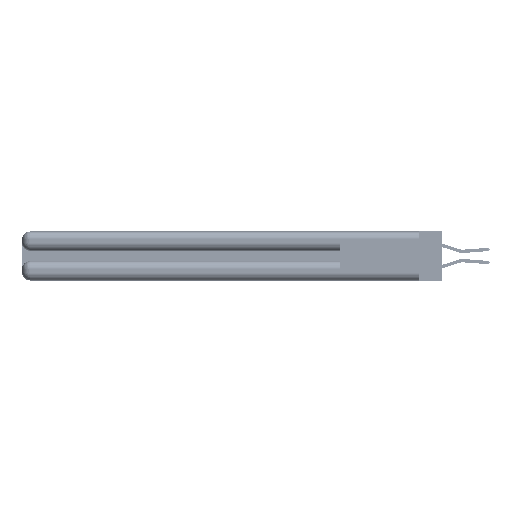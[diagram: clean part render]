
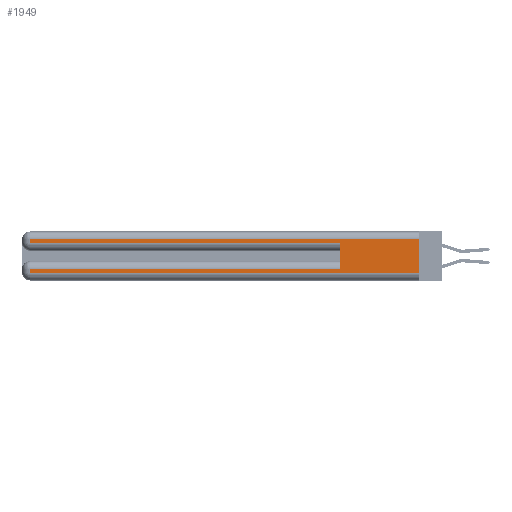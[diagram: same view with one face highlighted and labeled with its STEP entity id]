
A CAD part, left-side view. The second image highlights one B-rep face of the part: STEP entity #1949.
In plain terms, the highlighted planar face has unit normal (-1, 0, 0).
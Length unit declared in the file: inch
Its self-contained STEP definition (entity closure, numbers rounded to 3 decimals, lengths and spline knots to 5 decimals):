
#197 = VECTOR ( 'NONE', #21409, 39.37008 ) ;
#849 = CARTESIAN_POINT ( 'NONE',  ( 0., 0.6, 0.145 ) ) ;
#1949 = ADVANCED_FACE ( 'NONE', ( #14343 ), #17856, .F. ) ;
#2125 = CARTESIAN_POINT ( 'NONE',  ( 0., 0., 0.06 ) ) ;
#2189 = EDGE_CURVE ( 'NONE', #31588, #5667, #36107, .T. ) ;
#2326 = DIRECTION ( 'NONE',  ( 0., 0., -1. ) ) ;
#3190 = CARTESIAN_POINT ( 'NONE',  ( 0., 0., 0.31 ) ) ;
#3318 = EDGE_CURVE ( 'NONE', #8492, #39988, #34006, .T. ) ;
#4852 = AXIS2_PLACEMENT_3D ( 'NONE', #13588, #9310, #22088 ) ;
#4855 = VECTOR ( 'NONE', #26163, 39.37008 ) ;
#5667 = VERTEX_POINT ( 'NONE', #52385 ) ;
#6557 = EDGE_CURVE ( 'NONE', #14769, #17361, #39207, .T. ) ;
#6794 = EDGE_CURVE ( 'NONE', #20744, #17361, #37201, .T. ) ;
#6870 = LINE ( 'NONE', #19288, #27984 ) ;
#8383 = EDGE_CURVE ( 'NONE', #20744, #12990, #44927, .T. ) ;
#8492 = VERTEX_POINT ( 'NONE', #11783 ) ;
#9310 = DIRECTION ( 'NONE',  ( 1., 0., 0. ) ) ;
#9988 = LINE ( 'NONE', #36077, #31182 ) ;
#10097 = LINE ( 'NONE', #12913, #197 ) ;
#11430 = ORIENTED_EDGE ( 'NONE', *, *, #38793, .T. ) ;
#11783 = CARTESIAN_POINT ( 'NONE',  ( 0., 0., 0.31 ) ) ;
#12913 = CARTESIAN_POINT ( 'NONE',  ( 0., 2.94, 0.37 ) ) ;
#12958 = EDGE_CURVE ( 'NONE', #39988, #14769, #10097, .T. ) ;
#12990 = VERTEX_POINT ( 'NONE', #42606 ) ;
#13499 = ORIENTED_EDGE ( 'NONE', *, *, #2189, .T. ) ;
#13588 = CARTESIAN_POINT ( 'NONE',  ( 0., 0., 0.37 ) ) ;
#14061 = ORIENTED_EDGE ( 'NONE', *, *, #12958, .T. ) ;
#14343 = FACE_OUTER_BOUND ( 'NONE', #54278, .T. ) ;
#14769 = VERTEX_POINT ( 'NONE', #50677 ) ;
#15781 = CARTESIAN_POINT ( 'NONE',  ( 0., 2.94, 0.31 ) ) ;
#16213 = CARTESIAN_POINT ( 'NONE',  ( 0., 0., 0.285 ) ) ;
#17361 = VERTEX_POINT ( 'NONE', #48994 ) ;
#17856 = PLANE ( 'NONE',  #4852 ) ;
#19288 = CARTESIAN_POINT ( 'NONE',  ( 0., 2.94, 0.37 ) ) ;
#20197 = ORIENTED_EDGE ( 'NONE', *, *, #8383, .T. ) ;
#20744 = VERTEX_POINT ( 'NONE', #27229 ) ;
#21409 = DIRECTION ( 'NONE',  ( 0., 0., -1. ) ) ;
#22088 = DIRECTION ( 'NONE',  ( 0., 0., -1. ) ) ;
#23833 = DIRECTION ( 'NONE',  ( 0., 1., 0. ) ) ;
#26163 = DIRECTION ( 'NONE',  ( 0., 0., 1. ) ) ;
#27229 = CARTESIAN_POINT ( 'NONE',  ( 0., 0.6, 0.085 ) ) ;
#27741 = DIRECTION ( 'NONE',  ( 0., 0., -1. ) ) ;
#27984 = VECTOR ( 'NONE', #27741, 39.37008 ) ;
#28502 = DIRECTION ( 'NONE',  ( 0., 1., 0. ) ) ;
#31182 = VECTOR ( 'NONE', #2326, 39.37008 ) ;
#31588 = VERTEX_POINT ( 'NONE', #40047 ) ;
#34006 = LINE ( 'NONE', #3190, #43891 ) ;
#34038 = ORIENTED_EDGE ( 'NONE', *, *, #39861, .F. ) ;
#34566 = ORIENTED_EDGE ( 'NONE', *, *, #6794, .F. ) ;
#34798 = VECTOR ( 'NONE', #44369, 39.37008 ) ;
#36077 = CARTESIAN_POINT ( 'NONE',  ( 0., 0., 0.37 ) ) ;
#36107 = LINE ( 'NONE', #2125, #34798 ) ;
#36325 = CARTESIAN_POINT ( 'NONE',  ( 0., 0., 0.085 ) ) ;
#37201 = LINE ( 'NONE', #849, #4855 ) ;
#37884 = ORIENTED_EDGE ( 'NONE', *, *, #6557, .T. ) ;
#38614 = ORIENTED_EDGE ( 'NONE', *, *, #3318, .T. ) ;
#38793 = EDGE_CURVE ( 'NONE', #12990, #31588, #6870, .T. ) ;
#39207 = LINE ( 'NONE', #16213, #46468 ) ;
#39861 = EDGE_CURVE ( 'NONE', #8492, #5667, #9988, .T. ) ;
#39988 = VERTEX_POINT ( 'NONE', #15781 ) ;
#40047 = CARTESIAN_POINT ( 'NONE',  ( 0., 2.94, 0.06 ) ) ;
#42606 = CARTESIAN_POINT ( 'NONE',  ( 0., 2.94, 0.085 ) ) ;
#43608 = VECTOR ( 'NONE', #23833, 39.37008 ) ;
#43891 = VECTOR ( 'NONE', #28502, 39.37008 ) ;
#44369 = DIRECTION ( 'NONE',  ( 0., -1., 0. ) ) ;
#44927 = LINE ( 'NONE', #36325, #43608 ) ;
#46468 = VECTOR ( 'NONE', #54159, 39.37008 ) ;
#48994 = CARTESIAN_POINT ( 'NONE',  ( 0., 0.6, 0.285 ) ) ;
#50677 = CARTESIAN_POINT ( 'NONE',  ( 0., 2.94, 0.285 ) ) ;
#52385 = CARTESIAN_POINT ( 'NONE',  ( 0., 0., 0.06 ) ) ;
#54159 = DIRECTION ( 'NONE',  ( 0., -1., 0. ) ) ;
#54278 = EDGE_LOOP ( 'NONE', ( #34038, #38614, #14061, #37884, #34566, #20197, #11430, #13499 ) ) ;
